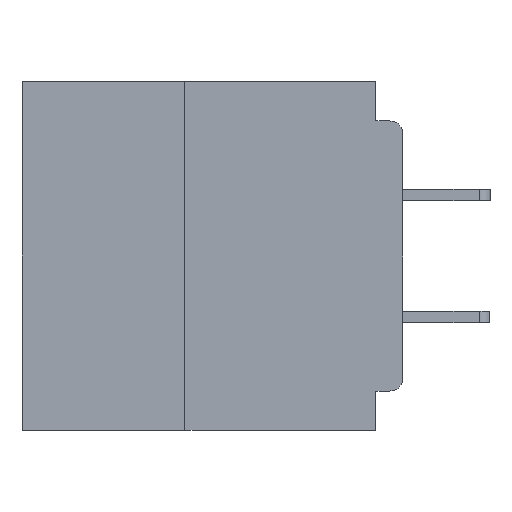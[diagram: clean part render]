
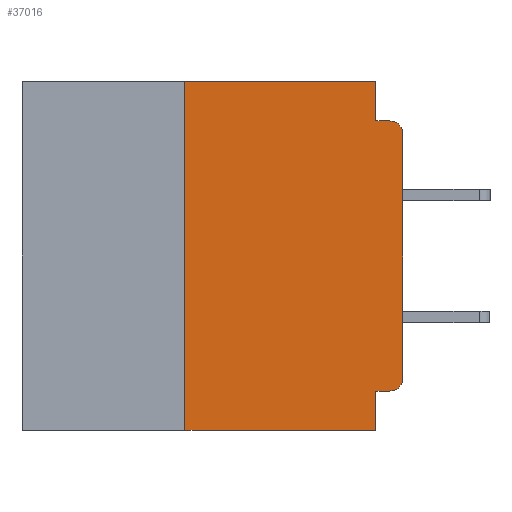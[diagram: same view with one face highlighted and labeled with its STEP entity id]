
A CAD part, left-side view. The second image highlights one B-rep face of the part: STEP entity #37016.
In plain terms, the highlighted planar face has unit normal (-1, 0, 0).
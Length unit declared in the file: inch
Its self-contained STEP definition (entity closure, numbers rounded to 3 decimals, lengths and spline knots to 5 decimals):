
#722 = CARTESIAN_POINT ( 'NONE',  ( 0., 0.031, -0.4 ) ) ;
#809 = CARTESIAN_POINT ( 'NONE',  ( 0., 0., -0.34 ) ) ;
#965 = EDGE_CURVE ( 'NONE', #20501, #47010, #3301, .T. ) ;
#1128 = EDGE_LOOP ( 'NONE', ( #32803, #33819, #35495, #37354, #38033, #39138, #41677, #43155, #44212, #45496 ) ) ;
#1281 = EDGE_CURVE ( 'NONE', #29486, #25682, #51560, .T. ) ;
#2019 = EDGE_CURVE ( 'NONE', #52314, #2660, #26148, .T. ) ;
#2347 = EDGE_CURVE ( 'NONE', #6902, #25682, #52078, .T. ) ;
#2381 = DIRECTION ( 'NONE',  ( 0., 1., 0. ) ) ;
#2502 = PLANE ( 'NONE',  #30749 ) ;
#2510 = VECTOR ( 'NONE', #39355, 39.37008 ) ;
#2660 = VERTEX_POINT ( 'NONE', #14418 ) ;
#3301 = CIRCLE ( 'NONE', #28691, 0.015 ) ;
#6888 = CARTESIAN_POINT ( 'NONE',  ( 0., 0.437, 0. ) ) ;
#6902 = VERTEX_POINT ( 'NONE', #15525 ) ;
#7110 = DIRECTION ( 'NONE',  ( -1., 0., 0. ) ) ;
#7187 = VECTOR ( 'NONE', #32105, 39.37008 ) ;
#7234 = DIRECTION ( 'NONE',  ( 0., 0., -1. ) ) ;
#7293 = CARTESIAN_POINT ( 'NONE',  ( 0., 0.015, -0.06 ) ) ;
#8846 = EDGE_CURVE ( 'NONE', #15707, #52314, #48151, .T. ) ;
#9528 = CARTESIAN_POINT ( 'NONE',  ( 0., 0.25, -0.4 ) ) ;
#9770 = DIRECTION ( 'NONE',  ( -1., 0., 0. ) ) ;
#11154 = CARTESIAN_POINT ( 'NONE',  ( 0., 0.437, 0. ) ) ;
#11174 = DIRECTION ( 'NONE',  ( 0., 0., -1. ) ) ;
#12566 = VERTEX_POINT ( 'NONE', #809 ) ;
#13235 = VECTOR ( 'NONE', #2381, 39.37008 ) ;
#13758 = DIRECTION ( 'NONE',  ( 0., 0., 1. ) ) ;
#13940 = DIRECTION ( 'NONE',  ( 0., 0., -1. ) ) ;
#14185 = CARTESIAN_POINT ( 'NONE',  ( 0., 0.031, -0.4 ) ) ;
#14418 = CARTESIAN_POINT ( 'NONE',  ( 0., 0.031, -0.045 ) ) ;
#14868 = CARTESIAN_POINT ( 'NONE',  ( 0., 0., -0.355 ) ) ;
#15525 = CARTESIAN_POINT ( 'NONE',  ( 0., 0.031, -0.355 ) ) ;
#15707 = VERTEX_POINT ( 'NONE', #19847 ) ;
#16333 = VERTEX_POINT ( 'NONE', #52650 ) ;
#17590 = LINE ( 'NONE', #31272, #27438 ) ;
#17702 = CIRCLE ( 'NONE', #22092, 0.015 ) ;
#19847 = CARTESIAN_POINT ( 'NONE',  ( 0., 0.25, 0. ) ) ;
#20501 = VERTEX_POINT ( 'NONE', #49717 ) ;
#22008 = FACE_OUTER_BOUND ( 'NONE', #1128, .T. ) ;
#22092 = AXIS2_PLACEMENT_3D ( 'NONE', #34859, #9770, #39036 ) ;
#23023 = DIRECTION ( 'NONE',  ( 0., 0., 1. ) ) ;
#25682 = VERTEX_POINT ( 'NONE', #722 ) ;
#26148 = LINE ( 'NONE', #45639, #2510 ) ;
#27438 = VECTOR ( 'NONE', #23023, 39.37008 ) ;
#28691 = AXIS2_PLACEMENT_3D ( 'NONE', #7293, #7110, #7234 ) ;
#29112 = EDGE_CURVE ( 'NONE', #16333, #6902, #35518, .T. ) ;
#29425 = EDGE_CURVE ( 'NONE', #29486, #15707, #30900, .T. ) ;
#29486 = VERTEX_POINT ( 'NONE', #43300 ) ;
#30144 = EDGE_CURVE ( 'NONE', #16333, #12566, #17702, .T. ) ;
#30749 = AXIS2_PLACEMENT_3D ( 'NONE', #6888, #36231, #11174 ) ;
#30900 = LINE ( 'NONE', #9528, #51617 ) ;
#31272 = CARTESIAN_POINT ( 'NONE',  ( 0., 0., 0. ) ) ;
#32030 = LINE ( 'NONE', #46745, #52715 ) ;
#32105 = DIRECTION ( 'NONE',  ( 0., -1., 0. ) ) ;
#32803 = ORIENTED_EDGE ( 'NONE', *, *, #35610, .T. ) ;
#33819 = ORIENTED_EDGE ( 'NONE', *, *, #965, .T. ) ;
#34859 = CARTESIAN_POINT ( 'NONE',  ( 0., 0.015, -0.34 ) ) ;
#35495 = ORIENTED_EDGE ( 'NONE', *, *, #50301, .F. ) ;
#35518 = LINE ( 'NONE', #14868, #13235 ) ;
#35610 = EDGE_CURVE ( 'NONE', #12566, #20501, #17590, .T. ) ;
#36231 = DIRECTION ( 'NONE',  ( 1., 0., 0. ) ) ;
#37016 = ADVANCED_FACE ( 'NONE', ( #22008 ), #2502, .F. ) ;
#37354 = ORIENTED_EDGE ( 'NONE', *, *, #2019, .F. ) ;
#38033 = ORIENTED_EDGE ( 'NONE', *, *, #8846, .F. ) ;
#39036 = DIRECTION ( 'NONE',  ( 0., 0., -1. ) ) ;
#39138 = ORIENTED_EDGE ( 'NONE', *, *, #29425, .F. ) ;
#39355 = DIRECTION ( 'NONE',  ( 0., 0., -1. ) ) ;
#40403 = DIRECTION ( 'NONE',  ( 0., -1., 0. ) ) ;
#41677 = ORIENTED_EDGE ( 'NONE', *, *, #1281, .T. ) ;
#43155 = ORIENTED_EDGE ( 'NONE', *, *, #2347, .F. ) ;
#43300 = CARTESIAN_POINT ( 'NONE',  ( 0., 0.25, -0.4 ) ) ;
#44212 = ORIENTED_EDGE ( 'NONE', *, *, #29112, .F. ) ;
#45496 = ORIENTED_EDGE ( 'NONE', *, *, #30144, .T. ) ;
#45639 = CARTESIAN_POINT ( 'NONE',  ( 0., 0.031, 0. ) ) ;
#46745 = CARTESIAN_POINT ( 'NONE',  ( 0., 0., -0.045 ) ) ;
#46832 = VECTOR ( 'NONE', #40403, 39.37008 ) ;
#47010 = VERTEX_POINT ( 'NONE', #48463 ) ;
#48151 = LINE ( 'NONE', #11154, #46832 ) ;
#48190 = CARTESIAN_POINT ( 'NONE',  ( 0., 0.031, 0. ) ) ;
#48463 = CARTESIAN_POINT ( 'NONE',  ( 0., 0.015, -0.045 ) ) ;
#49717 = CARTESIAN_POINT ( 'NONE',  ( 0., 0., -0.06 ) ) ;
#50301 = EDGE_CURVE ( 'NONE', #2660, #47010, #32030, .T. ) ;
#50901 = DIRECTION ( 'NONE',  ( 0., -1., 0. ) ) ;
#51129 = CARTESIAN_POINT ( 'NONE',  ( 0., 0.437, -0.4 ) ) ;
#51560 = LINE ( 'NONE', #51129, #7187 ) ;
#51617 = VECTOR ( 'NONE', #13758, 39.37008 ) ;
#52078 = LINE ( 'NONE', #14185, #53393 ) ;
#52314 = VERTEX_POINT ( 'NONE', #48190 ) ;
#52650 = CARTESIAN_POINT ( 'NONE',  ( 0., 0.015, -0.355 ) ) ;
#52715 = VECTOR ( 'NONE', #50901, 39.37008 ) ;
#53393 = VECTOR ( 'NONE', #13940, 39.37008 ) ;
